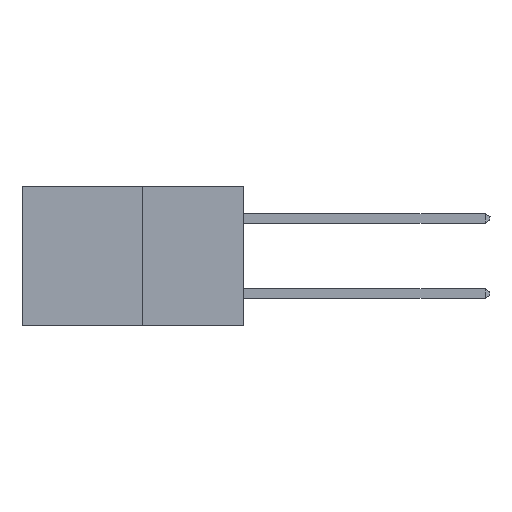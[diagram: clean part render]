
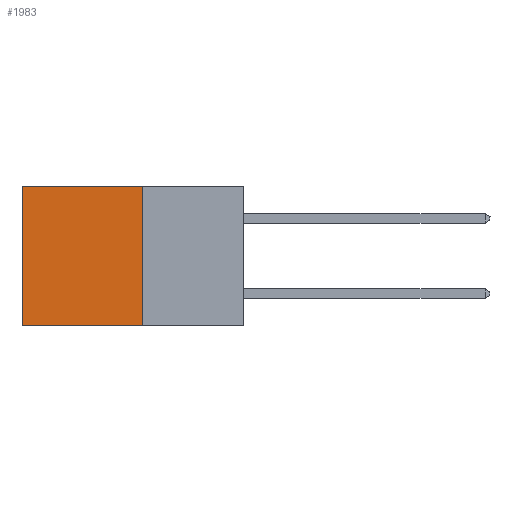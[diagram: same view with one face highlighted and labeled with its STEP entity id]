
A CAD part, left-side view. The second image highlights one B-rep face of the part: STEP entity #1983.
In plain terms, the highlighted planar face has unit normal (-1, 0, 0).
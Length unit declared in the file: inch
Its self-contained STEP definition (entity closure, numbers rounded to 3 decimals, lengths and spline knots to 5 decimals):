
#528 = VECTOR ( 'NONE', #18153, 39.37008 ) ;
#1012 = LINE ( 'NONE', #8607, #528 ) ;
#1260 = VERTEX_POINT ( 'NONE', #14765 ) ;
#1800 = CARTESIAN_POINT ( 'NONE',  ( 0.277, 0.59, -0.37 ) ) ;
#1983 = ADVANCED_FACE ( 'NONE', ( #20181 ), #5510, .F. ) ;
#2783 = CARTESIAN_POINT ( 'NONE',  ( 0.277, 0.27, 0. ) ) ;
#3156 = VECTOR ( 'NONE', #15939, 39.37008 ) ;
#3668 = LINE ( 'NONE', #19025, #3156 ) ;
#3861 = EDGE_CURVE ( 'NONE', #1260, #18900, #10037, .T. ) ;
#5363 = EDGE_CURVE ( 'NONE', #11368, #1260, #8303, .T. ) ;
#5510 = PLANE ( 'NONE',  #13090 ) ;
#7511 = ORIENTED_EDGE ( 'NONE', *, *, #13732, .F. ) ;
#7729 = EDGE_LOOP ( 'NONE', ( #10222, #7511, #20210, #8032 ) ) ;
#8032 = ORIENTED_EDGE ( 'NONE', *, *, #5363, .T. ) ;
#8303 = LINE ( 'NONE', #12113, #20359 ) ;
#8607 = CARTESIAN_POINT ( 'NONE',  ( 0.277, 0.27, -0.37 ) ) ;
#9900 = EDGE_CURVE ( 'NONE', #11368, #14327, #1012, .T. ) ;
#10037 = LINE ( 'NONE', #1800, #13722 ) ;
#10222 = ORIENTED_EDGE ( 'NONE', *, *, #3861, .T. ) ;
#11368 = VERTEX_POINT ( 'NONE', #2783 ) ;
#12026 = DIRECTION ( 'NONE',  ( 0., 1., 0. ) ) ;
#12113 = CARTESIAN_POINT ( 'NONE',  ( 0.277, 0.27, 0. ) ) ;
#13090 = AXIS2_PLACEMENT_3D ( 'NONE', #15716, #17023, #16993 ) ;
#13505 = CARTESIAN_POINT ( 'NONE',  ( 0.277, 0.59, -0.37 ) ) ;
#13722 = VECTOR ( 'NONE', #18685, 39.37008 ) ;
#13732 = EDGE_CURVE ( 'NONE', #14327, #18900, #3668, .T. ) ;
#13995 = CARTESIAN_POINT ( 'NONE',  ( 0.277, 0.27, -0.37 ) ) ;
#14327 = VERTEX_POINT ( 'NONE', #13995 ) ;
#14765 = CARTESIAN_POINT ( 'NONE',  ( 0.277, 0.59, 0. ) ) ;
#15716 = CARTESIAN_POINT ( 'NONE',  ( 0.277, 0.27, -0.37 ) ) ;
#15939 = DIRECTION ( 'NONE',  ( 0., 1., 0. ) ) ;
#16993 = DIRECTION ( 'NONE',  ( 0., 0., -1. ) ) ;
#17023 = DIRECTION ( 'NONE',  ( 1., 0., 0. ) ) ;
#18153 = DIRECTION ( 'NONE',  ( 0., 0., -1. ) ) ;
#18685 = DIRECTION ( 'NONE',  ( 0., 0., -1. ) ) ;
#18900 = VERTEX_POINT ( 'NONE', #13505 ) ;
#19025 = CARTESIAN_POINT ( 'NONE',  ( 0.277, 0.27, -0.37 ) ) ;
#20181 = FACE_OUTER_BOUND ( 'NONE', #7729, .T. ) ;
#20210 = ORIENTED_EDGE ( 'NONE', *, *, #9900, .F. ) ;
#20359 = VECTOR ( 'NONE', #12026, 39.37008 ) ;
